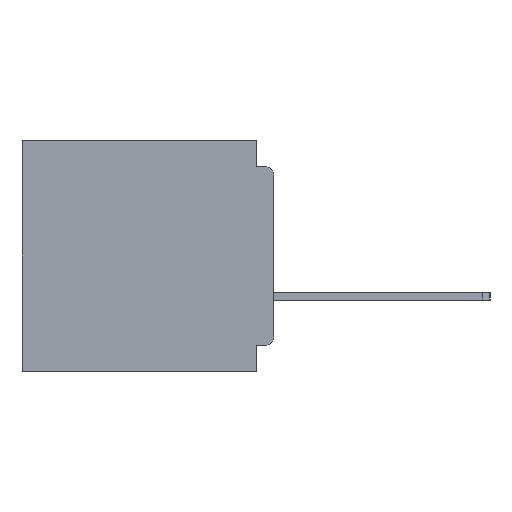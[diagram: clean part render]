
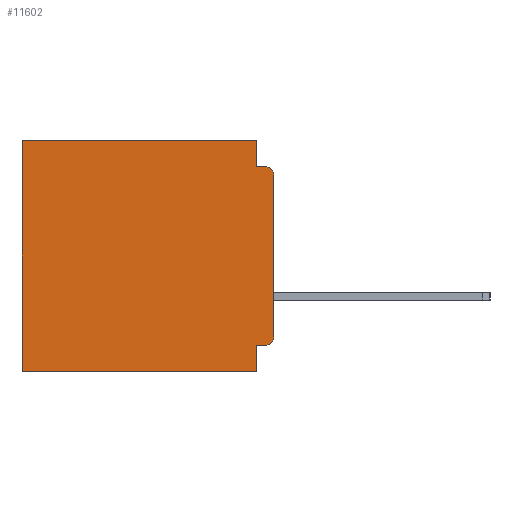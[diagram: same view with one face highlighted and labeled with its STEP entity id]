
A CAD part, left-side view. The second image highlights one B-rep face of the part: STEP entity #11602.
In plain terms, the highlighted planar face has unit normal (-1, 0, 0).
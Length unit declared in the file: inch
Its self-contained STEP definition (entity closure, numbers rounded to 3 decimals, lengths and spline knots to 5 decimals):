
#570 = VECTOR ( 'NONE', #8661, 39.37008 ) ;
#735 = LINE ( 'NONE', #5391, #33036 ) ;
#1073 = CARTESIAN_POINT ( 'NONE',  ( 0.3, 0.031, -0.4 ) ) ;
#1182 = CARTESIAN_POINT ( 'NONE',  ( 0.3, 0., -0.4 ) ) ;
#1516 = EDGE_LOOP ( 'NONE', ( #42791, #34497, #16888, #5470, #41442, #33749, #12462, #38017, #48626, #45747 ) ) ;
#2522 = VERTEX_POINT ( 'NONE', #42070 ) ;
#2549 = CARTESIAN_POINT ( 'NONE',  ( 0.3, 0., -0.4 ) ) ;
#4732 = CARTESIAN_POINT ( 'NONE',  ( 0.3, 0., -0.06 ) ) ;
#4739 = AXIS2_PLACEMENT_3D ( 'NONE', #30492, #6233, #34499 ) ;
#5239 = DIRECTION ( 'NONE',  ( 0., 1., 0. ) ) ;
#5261 = CARTESIAN_POINT ( 'NONE',  ( 0.3, 0.437, -0.4 ) ) ;
#5391 = CARTESIAN_POINT ( 'NONE',  ( 0.3, 0., 0. ) ) ;
#5470 = ORIENTED_EDGE ( 'NONE', *, *, #11288, .F. ) ;
#6233 = DIRECTION ( 'NONE',  ( -1., 0., 0. ) ) ;
#8392 = EDGE_CURVE ( 'NONE', #12518, #28965, #42179, .T. ) ;
#8661 = DIRECTION ( 'NONE',  ( 0., -1., 0. ) ) ;
#10466 = CARTESIAN_POINT ( 'NONE',  ( 0.3, 0.437, 0. ) ) ;
#10573 = VERTEX_POINT ( 'NONE', #5261 ) ;
#10608 = CARTESIAN_POINT ( 'NONE',  ( 0.3, 0.437, -0.4 ) ) ;
#10827 = LINE ( 'NONE', #44974, #39276 ) ;
#11288 = EDGE_CURVE ( 'NONE', #13550, #2522, #27060, .T. ) ;
#11351 = LINE ( 'NONE', #12733, #570 ) ;
#11602 = ADVANCED_FACE ( 'NONE', ( #21310 ), #30712, .F. ) ;
#11701 = CARTESIAN_POINT ( 'NONE',  ( 0.3, 0.015, -0.34 ) ) ;
#12462 = ORIENTED_EDGE ( 'NONE', *, *, #42569, .F. ) ;
#12518 = VERTEX_POINT ( 'NONE', #4732 ) ;
#12733 = CARTESIAN_POINT ( 'NONE',  ( 0.3, 0., -0.045 ) ) ;
#13031 = VERTEX_POINT ( 'NONE', #20865 ) ;
#13390 = CARTESIAN_POINT ( 'NONE',  ( 0.3, 0.015, -0.355 ) ) ;
#13550 = VERTEX_POINT ( 'NONE', #19909 ) ;
#13927 = VERTEX_POINT ( 'NONE', #10466 ) ;
#15544 = VERTEX_POINT ( 'NONE', #13390 ) ;
#15785 = DIRECTION ( 'NONE',  ( 0., 0., -1. ) ) ;
#16196 = CIRCLE ( 'NONE', #31022, 0.015 ) ;
#16273 = VECTOR ( 'NONE', #49005, 39.37008 ) ;
#16888 = ORIENTED_EDGE ( 'NONE', *, *, #23964, .F. ) ;
#18441 = DIRECTION ( 'NONE',  ( 0., 0., -1. ) ) ;
#19292 = EDGE_CURVE ( 'NONE', #15544, #26274, #10827, .T. ) ;
#19724 = VECTOR ( 'NONE', #5239, 39.37008 ) ;
#19909 = CARTESIAN_POINT ( 'NONE',  ( 0.3, 0.031, 0. ) ) ;
#20865 = CARTESIAN_POINT ( 'NONE',  ( 0.3, 0., -0.34 ) ) ;
#21310 = FACE_OUTER_BOUND ( 'NONE', #1516, .T. ) ;
#21680 = EDGE_CURVE ( 'NONE', #26274, #45811, #51018, .T. ) ;
#22937 = DIRECTION ( 'NONE',  ( 0., 0., -1. ) ) ;
#23964 = EDGE_CURVE ( 'NONE', #2522, #28965, #11351, .T. ) ;
#25125 = LINE ( 'NONE', #10608, #46510 ) ;
#26274 = VERTEX_POINT ( 'NONE', #45446 ) ;
#26666 = EDGE_CURVE ( 'NONE', #15544, #13031, #16196, .T. ) ;
#27060 = LINE ( 'NONE', #32847, #16273 ) ;
#28965 = VERTEX_POINT ( 'NONE', #29412 ) ;
#29412 = CARTESIAN_POINT ( 'NONE',  ( 0.3, 0.015, -0.045 ) ) ;
#29689 = AXIS2_PLACEMENT_3D ( 'NONE', #2549, #47035, #22937 ) ;
#30492 = CARTESIAN_POINT ( 'NONE',  ( 0.3, 0.015, -0.06 ) ) ;
#30712 = PLANE ( 'NONE',  #29689 ) ;
#31022 = AXIS2_PLACEMENT_3D ( 'NONE', #11701, #39951, #15785 ) ;
#32847 = CARTESIAN_POINT ( 'NONE',  ( 0.3, 0.031, 0. ) ) ;
#33036 = VECTOR ( 'NONE', #41812, 39.37008 ) ;
#33749 = ORIENTED_EDGE ( 'NONE', *, *, #36110, .T. ) ;
#34485 = CARTESIAN_POINT ( 'NONE',  ( 0.3, 0., -0.4 ) ) ;
#34497 = ORIENTED_EDGE ( 'NONE', *, *, #8392, .T. ) ;
#34499 = DIRECTION ( 'NONE',  ( 0., 0., -1. ) ) ;
#36095 = CARTESIAN_POINT ( 'NONE',  ( 0.3, 0.031, -0.4 ) ) ;
#36110 = EDGE_CURVE ( 'NONE', #13927, #10573, #25125, .T. ) ;
#37052 = DIRECTION ( 'NONE',  ( 0., 1., 0. ) ) ;
#38017 = ORIENTED_EDGE ( 'NONE', *, *, #21680, .F. ) ;
#38882 = DIRECTION ( 'NONE',  ( 0., 0., -1. ) ) ;
#39088 = VECTOR ( 'NONE', #40115, 39.37008 ) ;
#39276 = VECTOR ( 'NONE', #37052, 39.37008 ) ;
#39951 = DIRECTION ( 'NONE',  ( -1., 0., 0. ) ) ;
#40115 = DIRECTION ( 'NONE',  ( 0., 0., -1. ) ) ;
#40889 = VECTOR ( 'NONE', #18441, 39.37008 ) ;
#41165 = LINE ( 'NONE', #1182, #19724 ) ;
#41416 = EDGE_CURVE ( 'NONE', #13550, #13927, #735, .T. ) ;
#41442 = ORIENTED_EDGE ( 'NONE', *, *, #41416, .T. ) ;
#41812 = DIRECTION ( 'NONE',  ( 0., 1., 0. ) ) ;
#42070 = CARTESIAN_POINT ( 'NONE',  ( 0.3, 0.031, -0.045 ) ) ;
#42179 = CIRCLE ( 'NONE', #4739, 0.015 ) ;
#42569 = EDGE_CURVE ( 'NONE', #45811, #10573, #41165, .T. ) ;
#42791 = ORIENTED_EDGE ( 'NONE', *, *, #47736, .F. ) ;
#44974 = CARTESIAN_POINT ( 'NONE',  ( 0.3, 0., -0.355 ) ) ;
#45446 = CARTESIAN_POINT ( 'NONE',  ( 0.3, 0.031, -0.355 ) ) ;
#45747 = ORIENTED_EDGE ( 'NONE', *, *, #26666, .T. ) ;
#45811 = VERTEX_POINT ( 'NONE', #1073 ) ;
#46510 = VECTOR ( 'NONE', #38882, 39.37008 ) ;
#47035 = DIRECTION ( 'NONE',  ( 1., 0., 0. ) ) ;
#47736 = EDGE_CURVE ( 'NONE', #12518, #13031, #51575, .T. ) ;
#48626 = ORIENTED_EDGE ( 'NONE', *, *, #19292, .F. ) ;
#49005 = DIRECTION ( 'NONE',  ( 0., 0., -1. ) ) ;
#51018 = LINE ( 'NONE', #36095, #39088 ) ;
#51575 = LINE ( 'NONE', #34485, #40889 ) ;
